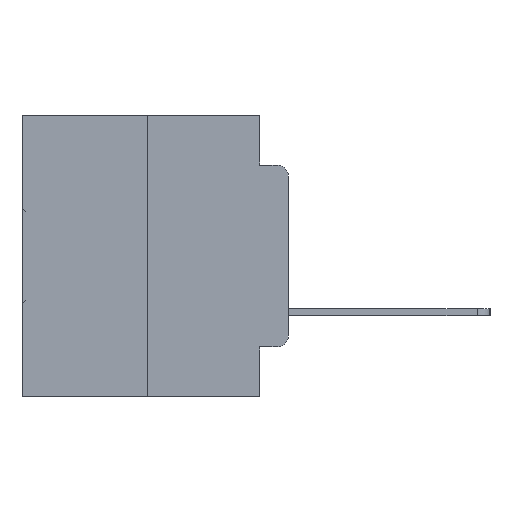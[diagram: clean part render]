
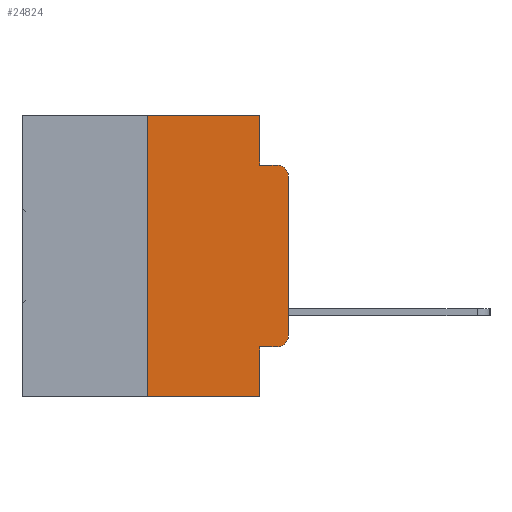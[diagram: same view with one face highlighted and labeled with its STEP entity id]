
A CAD part, left-side view. The second image highlights one B-rep face of the part: STEP entity #24824.
In plain terms, the highlighted planar face has unit normal (-1, 0, 0).
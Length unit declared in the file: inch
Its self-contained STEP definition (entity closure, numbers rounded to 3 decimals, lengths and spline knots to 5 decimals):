
#270 = CARTESIAN_POINT ( 'NONE',  ( 0., 0.051, 0. ) ) ;
#447 = VECTOR ( 'NONE', #10371, 39.37008 ) ;
#1040 = CARTESIAN_POINT ( 'NONE',  ( 0., 0., 0. ) ) ;
#1117 = LINE ( 'NONE', #23855, #14205 ) ;
#1129 = EDGE_CURVE ( 'NONE', #6833, #6125, #22759, .T. ) ;
#1247 = LINE ( 'NONE', #30742, #447 ) ;
#2048 = ORIENTED_EDGE ( 'NONE', *, *, #17087, .T. ) ;
#2112 = VECTOR ( 'NONE', #23841, 39.37008 ) ;
#2222 = CARTESIAN_POINT ( 'NONE',  ( 0., 0.02, -0.3915 ) ) ;
#2255 = CARTESIAN_POINT ( 'NONE',  ( 0., 0.051, 0. ) ) ;
#2358 = CARTESIAN_POINT ( 'NONE',  ( 0., 0., -0.3915 ) ) ;
#2857 = DIRECTION ( 'NONE',  ( 0., 0., -1. ) ) ;
#3042 = LINE ( 'NONE', #30725, #16125 ) ;
#3257 = DIRECTION ( 'NONE',  ( 0., -1., 0. ) ) ;
#4633 = VECTOR ( 'NONE', #3257, 39.37008 ) ;
#4858 = DIRECTION ( 'NONE',  ( 0., 0., -1. ) ) ;
#4871 = CARTESIAN_POINT ( 'NONE',  ( 0., 0.25, -0.5 ) ) ;
#4923 = AXIS2_PLACEMENT_3D ( 'NONE', #2222, #20411, #4858 ) ;
#5307 = EDGE_CURVE ( 'NONE', #6125, #26248, #16116, .T. ) ;
#5337 = CARTESIAN_POINT ( 'NONE',  ( 0., 0.25, 0. ) ) ;
#5376 = ORIENTED_EDGE ( 'NONE', *, *, #28989, .F. ) ;
#5435 = LINE ( 'NONE', #16171, #4633 ) ;
#5512 = DIRECTION ( 'NONE',  ( 1., 0., 0. ) ) ;
#6125 = VERTEX_POINT ( 'NONE', #24912 ) ;
#6266 = VERTEX_POINT ( 'NONE', #4871 ) ;
#6833 = VERTEX_POINT ( 'NONE', #27661 ) ;
#6904 = CARTESIAN_POINT ( 'NONE',  ( 0., 0.02, -0.0885 ) ) ;
#6916 = VERTEX_POINT ( 'NONE', #10266 ) ;
#7594 = ORIENTED_EDGE ( 'NONE', *, *, #5307, .T. ) ;
#8609 = CARTESIAN_POINT ( 'NONE',  ( 0., 0.02, -0.1085 ) ) ;
#9138 = ORIENTED_EDGE ( 'NONE', *, *, #12027, .F. ) ;
#10245 = EDGE_CURVE ( 'NONE', #12434, #6916, #1247, .T. ) ;
#10266 = CARTESIAN_POINT ( 'NONE',  ( 0., 0.051, -0.0885 ) ) ;
#10371 = DIRECTION ( 'NONE',  ( 0., 0., -1. ) ) ;
#11249 = DIRECTION ( 'NONE',  ( 0., 0., -1. ) ) ;
#11514 = VECTOR ( 'NONE', #29386, 39.37008 ) ;
#12027 = EDGE_CURVE ( 'NONE', #15000, #12434, #1117, .T. ) ;
#12434 = VERTEX_POINT ( 'NONE', #2255 ) ;
#12720 = AXIS2_PLACEMENT_3D ( 'NONE', #18507, #5512, #23550 ) ;
#13257 = DIRECTION ( 'NONE',  ( 0., 0., 1. ) ) ;
#13325 = PLANE ( 'NONE',  #12720 ) ;
#14205 = VECTOR ( 'NONE', #26413, 39.37008 ) ;
#14396 = EDGE_CURVE ( 'NONE', #6266, #15000, #14412, .T. ) ;
#14412 = LINE ( 'NONE', #5337, #33049 ) ;
#14607 = CARTESIAN_POINT ( 'NONE',  ( 0., 0.051, -0.4115 ) ) ;
#14839 = ORIENTED_EDGE ( 'NONE', *, *, #27529, .T. ) ;
#15000 = VERTEX_POINT ( 'NONE', #27954 ) ;
#15346 = EDGE_LOOP ( 'NONE', ( #15530, #2048, #5376, #16431, #9138, #24348, #14839, #26398, #17351, #7594 ) ) ;
#15530 = ORIENTED_EDGE ( 'NONE', *, *, #23786, .T. ) ;
#16116 = CIRCLE ( 'NONE', #4923, 0.02 ) ;
#16125 = VECTOR ( 'NONE', #33236, 39.37008 ) ;
#16171 = CARTESIAN_POINT ( 'NONE',  ( 0., 0.051, -0.0885 ) ) ;
#16431 = ORIENTED_EDGE ( 'NONE', *, *, #10245, .F. ) ;
#17087 = EDGE_CURVE ( 'NONE', #33053, #31136, #25786, .T. ) ;
#17351 = ORIENTED_EDGE ( 'NONE', *, *, #1129, .T. ) ;
#17511 = AXIS2_PLACEMENT_3D ( 'NONE', #8609, #26504, #11249 ) ;
#17629 = CARTESIAN_POINT ( 'NONE',  ( 0., 0.051, -0.5 ) ) ;
#17992 = VECTOR ( 'NONE', #2857, 39.37008 ) ;
#18372 = LINE ( 'NONE', #1040, #11514 ) ;
#18507 = CARTESIAN_POINT ( 'NONE',  ( 0., 0.473, 0. ) ) ;
#18783 = LINE ( 'NONE', #270, #17992 ) ;
#20411 = DIRECTION ( 'NONE',  ( -1., 0., 0. ) ) ;
#22759 = LINE ( 'NONE', #14607, #2112 ) ;
#23550 = DIRECTION ( 'NONE',  ( 0., 0., -1. ) ) ;
#23580 = EDGE_CURVE ( 'NONE', #6833, #24599, #18783, .T. ) ;
#23786 = EDGE_CURVE ( 'NONE', #26248, #33053, #18372, .T. ) ;
#23841 = DIRECTION ( 'NONE',  ( 0., -1., 0. ) ) ;
#23855 = CARTESIAN_POINT ( 'NONE',  ( 0., 0.473, 0. ) ) ;
#24348 = ORIENTED_EDGE ( 'NONE', *, *, #14396, .F. ) ;
#24599 = VERTEX_POINT ( 'NONE', #17629 ) ;
#24824 = ADVANCED_FACE ( 'NONE', ( #25403 ), #13325, .F. ) ;
#24912 = CARTESIAN_POINT ( 'NONE',  ( 0., 0.02, -0.4115 ) ) ;
#25403 = FACE_OUTER_BOUND ( 'NONE', #15346, .T. ) ;
#25786 = CIRCLE ( 'NONE', #17511, 0.02 ) ;
#26248 = VERTEX_POINT ( 'NONE', #2358 ) ;
#26398 = ORIENTED_EDGE ( 'NONE', *, *, #23580, .F. ) ;
#26413 = DIRECTION ( 'NONE',  ( 0., -1., 0. ) ) ;
#26504 = DIRECTION ( 'NONE',  ( -1., 0., 0. ) ) ;
#27529 = EDGE_CURVE ( 'NONE', #6266, #24599, #3042, .T. ) ;
#27661 = CARTESIAN_POINT ( 'NONE',  ( 0., 0.051, -0.4115 ) ) ;
#27954 = CARTESIAN_POINT ( 'NONE',  ( 0., 0.25, 0. ) ) ;
#28989 = EDGE_CURVE ( 'NONE', #6916, #31136, #5435, .T. ) ;
#29386 = DIRECTION ( 'NONE',  ( 0., 0., 1. ) ) ;
#30468 = CARTESIAN_POINT ( 'NONE',  ( 0., 0., -0.1085 ) ) ;
#30725 = CARTESIAN_POINT ( 'NONE',  ( 0., 0.473, -0.5 ) ) ;
#30742 = CARTESIAN_POINT ( 'NONE',  ( 0., 0.051, 0. ) ) ;
#31136 = VERTEX_POINT ( 'NONE', #6904 ) ;
#33049 = VECTOR ( 'NONE', #13257, 39.37008 ) ;
#33053 = VERTEX_POINT ( 'NONE', #30468 ) ;
#33236 = DIRECTION ( 'NONE',  ( 0., -1., 0. ) ) ;
